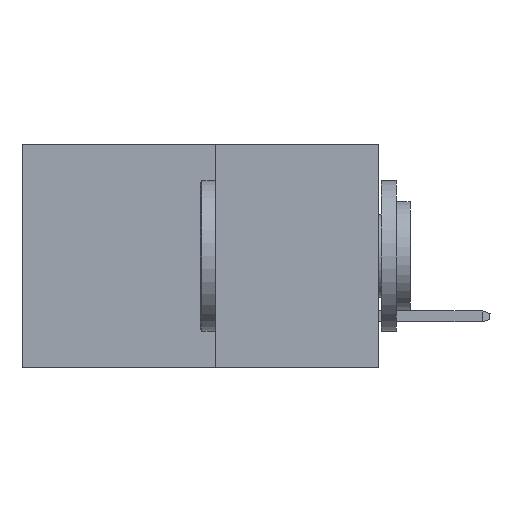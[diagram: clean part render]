
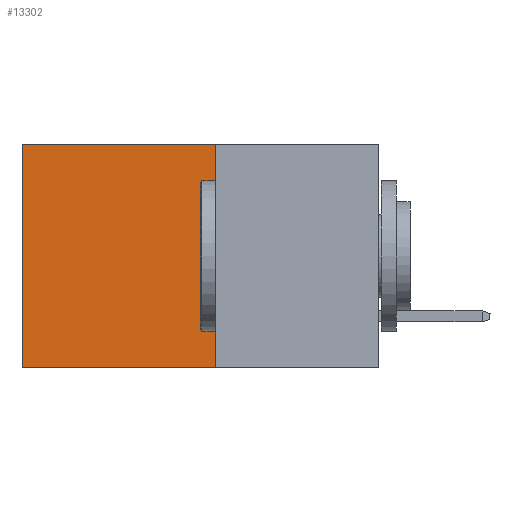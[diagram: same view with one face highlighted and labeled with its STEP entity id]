
A CAD part, left-side view. The second image highlights one B-rep face of the part: STEP entity #13302.
In plain terms, the highlighted planar face has unit normal (-1, 0, 0).
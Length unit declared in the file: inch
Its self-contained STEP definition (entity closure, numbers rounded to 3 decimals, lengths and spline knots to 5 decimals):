
#282 = DIRECTION ( 'NONE',  ( 0., 0., -1. ) ) ;
#435 = CARTESIAN_POINT ( 'NONE',  ( 0.277, 0.27, -0.37 ) ) ;
#872 = CARTESIAN_POINT ( 'NONE',  ( 0.277, 0.27, -0.37 ) ) ;
#910 = VERTEX_POINT ( 'NONE', #22716 ) ;
#936 = FACE_OUTER_BOUND ( 'NONE', #20373, .T. ) ;
#984 = CARTESIAN_POINT ( 'NONE',  ( 0.277, 0.59, 0. ) ) ;
#1735 = ORIENTED_EDGE ( 'NONE', *, *, #6568, .F. ) ;
#2639 = CARTESIAN_POINT ( 'NONE',  ( 0.277, 0.27, -0.37 ) ) ;
#2778 = VECTOR ( 'NONE', #282, 39.37008 ) ;
#4189 = LINE ( 'NONE', #24524, #21745 ) ;
#5920 = LINE ( 'NONE', #872, #16680 ) ;
#6568 = EDGE_CURVE ( 'NONE', #21982, #910, #14357, .T. ) ;
#7350 = DIRECTION ( 'NONE',  ( 0., 0., -1. ) ) ;
#7601 = ORIENTED_EDGE ( 'NONE', *, *, #14274, .T. ) ;
#9537 = ORIENTED_EDGE ( 'NONE', *, *, #9651, .F. ) ;
#9651 = EDGE_CURVE ( 'NONE', #910, #19468, #5920, .T. ) ;
#13302 = ADVANCED_FACE ( 'NONE', ( #936 ), #14170, .F. ) ;
#14170 = PLANE ( 'NONE',  #16407 ) ;
#14274 = EDGE_CURVE ( 'NONE', #29209, #19468, #4189, .T. ) ;
#14357 = LINE ( 'NONE', #435, #2778 ) ;
#16303 = LINE ( 'NONE', #22454, #26910 ) ;
#16407 = AXIS2_PLACEMENT_3D ( 'NONE', #2639, #20997, #7350 ) ;
#16680 = VECTOR ( 'NONE', #19319, 39.37008 ) ;
#18166 = CARTESIAN_POINT ( 'NONE',  ( 0.277, 0.59, -0.37 ) ) ;
#19319 = DIRECTION ( 'NONE',  ( 0., 1., 0. ) ) ;
#19468 = VERTEX_POINT ( 'NONE', #18166 ) ;
#20135 = ORIENTED_EDGE ( 'NONE', *, *, #21566, .T. ) ;
#20373 = EDGE_LOOP ( 'NONE', ( #7601, #9537, #1735, #20135 ) ) ;
#20997 = DIRECTION ( 'NONE',  ( 1., 0., 0. ) ) ;
#21566 = EDGE_CURVE ( 'NONE', #21982, #29209, #16303, .T. ) ;
#21745 = VECTOR ( 'NONE', #29035, 39.37008 ) ;
#21982 = VERTEX_POINT ( 'NONE', #26466 ) ;
#22454 = CARTESIAN_POINT ( 'NONE',  ( 0.277, 0.27, 0. ) ) ;
#22716 = CARTESIAN_POINT ( 'NONE',  ( 0.277, 0.27, -0.37 ) ) ;
#24524 = CARTESIAN_POINT ( 'NONE',  ( 0.277, 0.59, -0.37 ) ) ;
#24622 = DIRECTION ( 'NONE',  ( 0., 1., 0. ) ) ;
#26466 = CARTESIAN_POINT ( 'NONE',  ( 0.277, 0.27, 0. ) ) ;
#26910 = VECTOR ( 'NONE', #24622, 39.37008 ) ;
#29035 = DIRECTION ( 'NONE',  ( 0., 0., -1. ) ) ;
#29209 = VERTEX_POINT ( 'NONE', #984 ) ;
